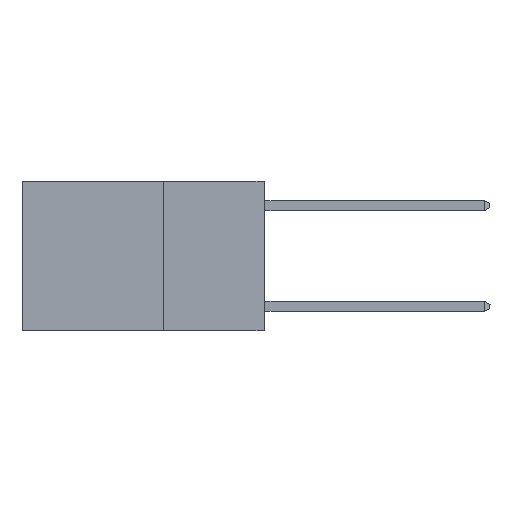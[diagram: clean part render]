
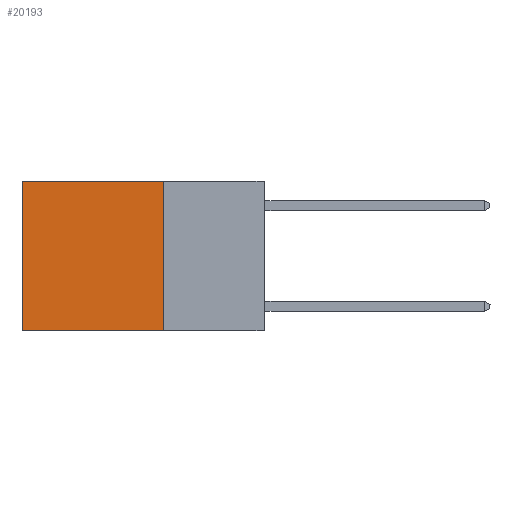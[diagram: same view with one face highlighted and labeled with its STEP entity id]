
A CAD part, left-side view. The second image highlights one B-rep face of the part: STEP entity #20193.
In plain terms, the highlighted planar face has unit normal (-1, 0, 0).
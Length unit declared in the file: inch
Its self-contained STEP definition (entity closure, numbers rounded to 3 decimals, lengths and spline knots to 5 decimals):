
#4 = ORIENTED_EDGE ( 'NONE', *, *, #16140, .T. ) ;
#7 = VERTEX_POINT ( 'NONE', #9919 ) ;
#451 = CARTESIAN_POINT ( 'NONE',  ( 0.2625, 0.6, 0. ) ) ;
#1020 = VERTEX_POINT ( 'NONE', #20444 ) ;
#1441 = CARTESIAN_POINT ( 'NONE',  ( 0.2625, 0.6, -0.37 ) ) ;
#1912 = DIRECTION ( 'NONE',  ( 0., 0., -1. ) ) ;
#1939 = VERTEX_POINT ( 'NONE', #1441 ) ;
#1999 = VERTEX_POINT ( 'NONE', #11140 ) ;
#2315 = LINE ( 'NONE', #4376, #22496 ) ;
#4376 = CARTESIAN_POINT ( 'NONE',  ( 0.2625, 0.25, -0.37 ) ) ;
#4866 = DIRECTION ( 'NONE',  ( 0., 1., 0. ) ) ;
#5781 = EDGE_LOOP ( 'NONE', ( #4, #16549, #7097, #23380 ) ) ;
#6155 = LINE ( 'NONE', #10589, #11390 ) ;
#7097 = ORIENTED_EDGE ( 'NONE', *, *, #24001, .F. ) ;
#7169 = VECTOR ( 'NONE', #4866, 39.37008 ) ;
#8217 = EDGE_CURVE ( 'NONE', #1999, #1020, #12387, .T. ) ;
#8734 = CARTESIAN_POINT ( 'NONE',  ( 0.2625, 0.25, 0. ) ) ;
#9772 = PLANE ( 'NONE',  #11473 ) ;
#9919 = CARTESIAN_POINT ( 'NONE',  ( 0.2625, 0.25, -0.37 ) ) ;
#10310 = DIRECTION ( 'NONE',  ( 0., 1., 0. ) ) ;
#10589 = CARTESIAN_POINT ( 'NONE',  ( 0.2625, 0.25, 0. ) ) ;
#11140 = CARTESIAN_POINT ( 'NONE',  ( 0.2625, 0.25, 0. ) ) ;
#11273 = LINE ( 'NONE', #451, #15848 ) ;
#11390 = VECTOR ( 'NONE', #24179, 39.37008 ) ;
#11473 = AXIS2_PLACEMENT_3D ( 'NONE', #25326, #13700, #1912 ) ;
#12387 = LINE ( 'NONE', #8734, #7169 ) ;
#13700 = DIRECTION ( 'NONE',  ( 1., 0., 0. ) ) ;
#15848 = VECTOR ( 'NONE', #18169, 39.37008 ) ;
#16140 = EDGE_CURVE ( 'NONE', #1020, #1939, #11273, .T. ) ;
#16549 = ORIENTED_EDGE ( 'NONE', *, *, #19688, .F. ) ;
#16733 = FACE_OUTER_BOUND ( 'NONE', #5781, .T. ) ;
#18169 = DIRECTION ( 'NONE',  ( 0., 0., -1. ) ) ;
#19688 = EDGE_CURVE ( 'NONE', #7, #1939, #2315, .T. ) ;
#20193 = ADVANCED_FACE ( 'NONE', ( #16733 ), #9772, .F. ) ;
#20444 = CARTESIAN_POINT ( 'NONE',  ( 0.2625, 0.6, 0. ) ) ;
#22496 = VECTOR ( 'NONE', #10310, 39.37008 ) ;
#23380 = ORIENTED_EDGE ( 'NONE', *, *, #8217, .T. ) ;
#24001 = EDGE_CURVE ( 'NONE', #1999, #7, #6155, .T. ) ;
#24179 = DIRECTION ( 'NONE',  ( 0., 0., -1. ) ) ;
#25326 = CARTESIAN_POINT ( 'NONE',  ( 0.2625, 0.25, 0. ) ) ;
